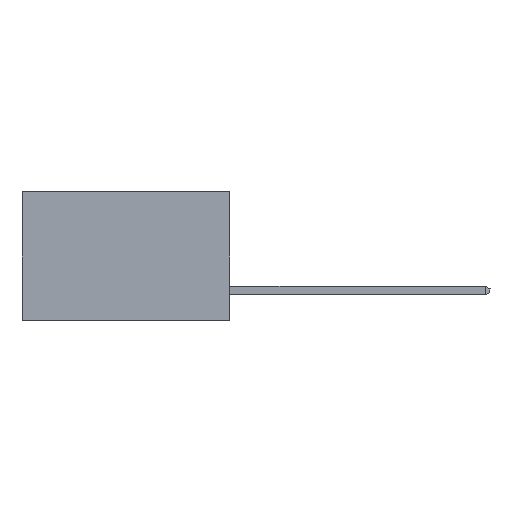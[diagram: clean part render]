
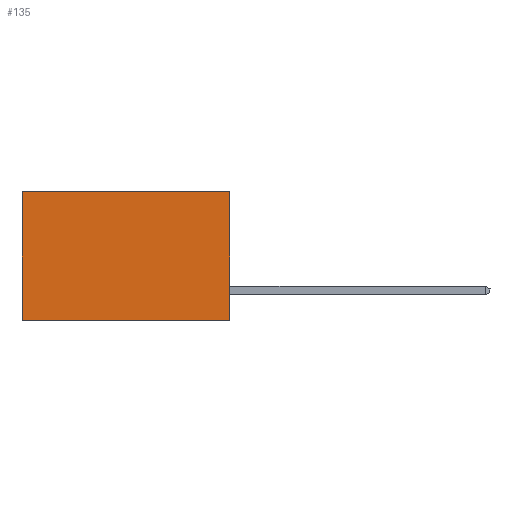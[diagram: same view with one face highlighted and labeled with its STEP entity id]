
A CAD part, left-side view. The second image highlights one B-rep face of the part: STEP entity #135.
In plain terms, the highlighted planar face has unit normal (-1, 0, 0).
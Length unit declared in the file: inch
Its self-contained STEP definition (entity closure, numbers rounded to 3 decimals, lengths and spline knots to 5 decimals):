
#135 = ADVANCED_FACE ( 'NONE', ( #10832 ), #2406, .F. ) ;
#474 = AXIS2_PLACEMENT_3D ( 'NONE', #4484, #10891, #8103 ) ;
#1481 = VERTEX_POINT ( 'NONE', #3536 ) ;
#1734 = DIRECTION ( 'NONE',  ( 0., 1., 0. ) ) ;
#1852 = EDGE_CURVE ( 'NONE', #4804, #6501, #6897, .T. ) ;
#1995 = EDGE_CURVE ( 'NONE', #7913, #1481, #9889, .T. ) ;
#2406 = PLANE ( 'NONE',  #474 ) ;
#3536 = CARTESIAN_POINT ( 'NONE',  ( 0.2615, 0.6, -0.37 ) ) ;
#3540 = CARTESIAN_POINT ( 'NONE',  ( 0.2615, 0.6, -0.37 ) ) ;
#3768 = VECTOR ( 'NONE', #5530, 39.37008 ) ;
#4237 = CARTESIAN_POINT ( 'NONE',  ( 0.2615, 0., 0. ) ) ;
#4484 = CARTESIAN_POINT ( 'NONE',  ( 0.2615, 0., -0.37 ) ) ;
#4488 = CARTESIAN_POINT ( 'NONE',  ( 0.2615, 0., -0.37 ) ) ;
#4682 = VECTOR ( 'NONE', #5316, 39.37008 ) ;
#4693 = CARTESIAN_POINT ( 'NONE',  ( 0.2615, 0., 0. ) ) ;
#4804 = VERTEX_POINT ( 'NONE', #4693 ) ;
#5198 = EDGE_CURVE ( 'NONE', #6501, #1481, #8949, .T. ) ;
#5316 = DIRECTION ( 'NONE',  ( 0., 1., 0. ) ) ;
#5530 = DIRECTION ( 'NONE',  ( 0., 0., -1. ) ) ;
#5713 = CARTESIAN_POINT ( 'NONE',  ( 0.2615, 0., -0.37 ) ) ;
#6501 = VERTEX_POINT ( 'NONE', #8424 ) ;
#6784 = ORIENTED_EDGE ( 'NONE', *, *, #1852, .T. ) ;
#6897 = LINE ( 'NONE', #4237, #4682 ) ;
#7913 = VERTEX_POINT ( 'NONE', #5713 ) ;
#8103 = DIRECTION ( 'NONE',  ( 0., 0., -1. ) ) ;
#8189 = ORIENTED_EDGE ( 'NONE', *, *, #1995, .F. ) ;
#8424 = CARTESIAN_POINT ( 'NONE',  ( 0.2615, 0.6, 0. ) ) ;
#8451 = VECTOR ( 'NONE', #1734, 39.37008 ) ;
#8949 = LINE ( 'NONE', #3540, #10186 ) ;
#9010 = DIRECTION ( 'NONE',  ( 0., 0., -1. ) ) ;
#9257 = LINE ( 'NONE', #9378, #3768 ) ;
#9378 = CARTESIAN_POINT ( 'NONE',  ( 0.2615, 0., -0.37 ) ) ;
#9692 = EDGE_LOOP ( 'NONE', ( #11514, #8189, #10727, #6784 ) ) ;
#9799 = EDGE_CURVE ( 'NONE', #4804, #7913, #9257, .T. ) ;
#9889 = LINE ( 'NONE', #4488, #8451 ) ;
#10186 = VECTOR ( 'NONE', #9010, 39.37008 ) ;
#10727 = ORIENTED_EDGE ( 'NONE', *, *, #9799, .F. ) ;
#10832 = FACE_OUTER_BOUND ( 'NONE', #9692, .T. ) ;
#10891 = DIRECTION ( 'NONE',  ( 1., 0., 0. ) ) ;
#11514 = ORIENTED_EDGE ( 'NONE', *, *, #5198, .T. ) ;
